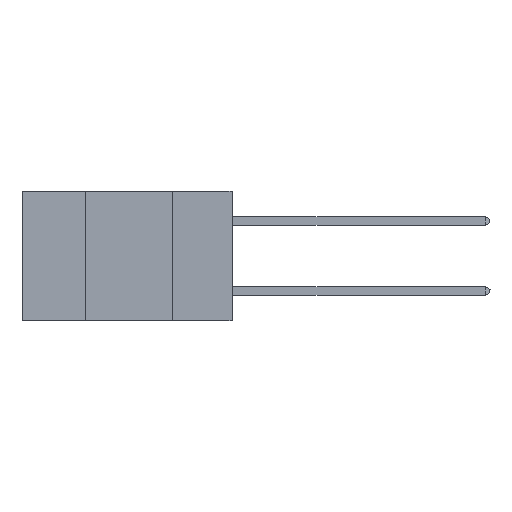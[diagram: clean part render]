
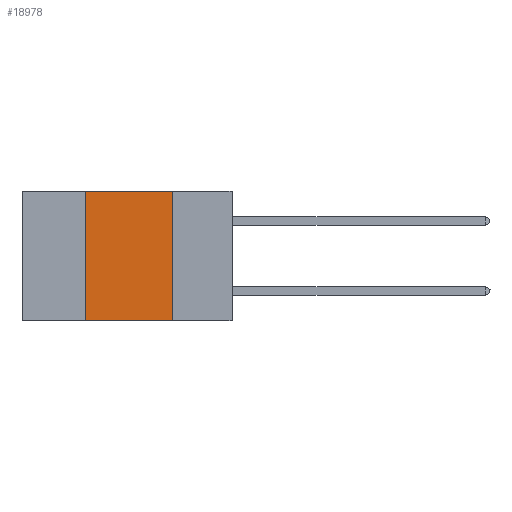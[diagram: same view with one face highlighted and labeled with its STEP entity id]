
A CAD part, left-side view. The second image highlights one B-rep face of the part: STEP entity #18978.
In plain terms, the highlighted planar face has unit normal (-1, 0, 0).
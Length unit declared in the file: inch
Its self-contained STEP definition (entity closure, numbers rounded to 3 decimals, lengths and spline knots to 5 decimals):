
#1285 = AXIS2_PLACEMENT_3D ( 'NONE', #11858, #14780, #34953 ) ;
#1915 = CARTESIAN_POINT ( 'NONE',  ( 0., 0.42, 0. ) ) ;
#2054 = EDGE_CURVE ( 'NONE', #29969, #6284, #18003, .T. ) ;
#4646 = VECTOR ( 'NONE', #8173, 39.37008 ) ;
#5255 = EDGE_CURVE ( 'NONE', #8825, #30082, #25351, .T. ) ;
#5363 = CARTESIAN_POINT ( 'NONE',  ( 0., 0.6, -0.37 ) ) ;
#6284 = VERTEX_POINT ( 'NONE', #1915 ) ;
#6562 = ORIENTED_EDGE ( 'NONE', *, *, #18393, .F. ) ;
#6646 = CARTESIAN_POINT ( 'NONE',  ( 0., 0.17, -0.37 ) ) ;
#6687 = EDGE_LOOP ( 'NONE', ( #11962, #6562, #30036, #8128 ) ) ;
#8128 = ORIENTED_EDGE ( 'NONE', *, *, #26193, .T. ) ;
#8173 = DIRECTION ( 'NONE',  ( 0., -1., 0. ) ) ;
#8263 = VECTOR ( 'NONE', #15550, 39.37008 ) ;
#8825 = VERTEX_POINT ( 'NONE', #33720 ) ;
#8897 = PLANE ( 'NONE',  #1285 ) ;
#11858 = CARTESIAN_POINT ( 'NONE',  ( 0., 0.6, 0. ) ) ;
#11962 = ORIENTED_EDGE ( 'NONE', *, *, #5255, .F. ) ;
#13181 = DIRECTION ( 'NONE',  ( 0., 0., 1. ) ) ;
#14780 = DIRECTION ( 'NONE',  ( 1., 0., 0. ) ) ;
#14843 = CARTESIAN_POINT ( 'NONE',  ( 0., 0.42, -0.37 ) ) ;
#15423 = CARTESIAN_POINT ( 'NONE',  ( 0., 0.6, 0. ) ) ;
#15550 = DIRECTION ( 'NONE',  ( 0., -1., 0. ) ) ;
#16043 = LINE ( 'NONE', #15423, #8263 ) ;
#18003 = LINE ( 'NONE', #27592, #32467 ) ;
#18393 = EDGE_CURVE ( 'NONE', #6284, #8825, #16043, .T. ) ;
#18978 = ADVANCED_FACE ( 'NONE', ( #25102 ), #8897, .F. ) ;
#21143 = CARTESIAN_POINT ( 'NONE',  ( 0., 0.17, 0. ) ) ;
#24045 = DIRECTION ( 'NONE',  ( 0., 0., -1. ) ) ;
#25102 = FACE_OUTER_BOUND ( 'NONE', #6687, .T. ) ;
#25351 = LINE ( 'NONE', #21143, #33019 ) ;
#26193 = EDGE_CURVE ( 'NONE', #29969, #30082, #35456, .T. ) ;
#27592 = CARTESIAN_POINT ( 'NONE',  ( 0., 0.42, 0. ) ) ;
#29969 = VERTEX_POINT ( 'NONE', #14843 ) ;
#30036 = ORIENTED_EDGE ( 'NONE', *, *, #2054, .F. ) ;
#30082 = VERTEX_POINT ( 'NONE', #6646 ) ;
#32467 = VECTOR ( 'NONE', #13181, 39.37008 ) ;
#33019 = VECTOR ( 'NONE', #24045, 39.37008 ) ;
#33720 = CARTESIAN_POINT ( 'NONE',  ( 0., 0.17, 0. ) ) ;
#34953 = DIRECTION ( 'NONE',  ( 0., 0., -1. ) ) ;
#35456 = LINE ( 'NONE', #5363, #4646 ) ;
